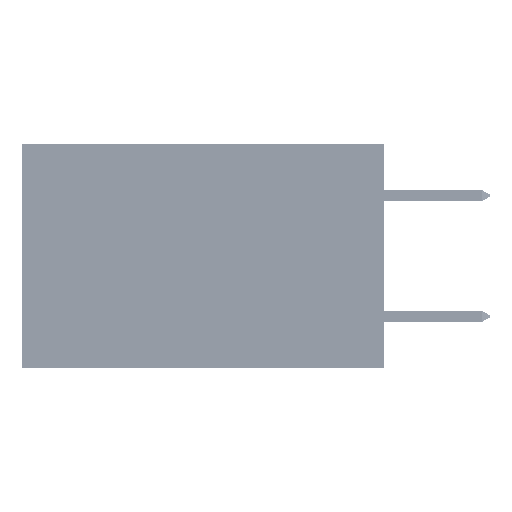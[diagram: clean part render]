
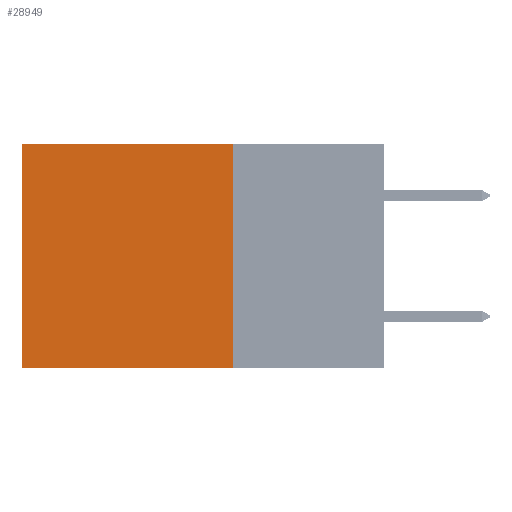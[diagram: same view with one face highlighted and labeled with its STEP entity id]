
A CAD part, left-side view. The second image highlights one B-rep face of the part: STEP entity #28949.
In plain terms, the highlighted planar face has unit normal (-1, 0, 0).
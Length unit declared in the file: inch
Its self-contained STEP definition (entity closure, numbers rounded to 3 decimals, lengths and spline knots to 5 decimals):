
#230 = VERTEX_POINT ( 'NONE', #17198 ) ;
#1277 = DIRECTION ( 'NONE',  ( 0., 0., -1. ) ) ;
#2487 = LINE ( 'NONE', #6239, #3672 ) ;
#3648 = VERTEX_POINT ( 'NONE', #31756 ) ;
#3672 = VECTOR ( 'NONE', #28453, 39.37008 ) ;
#4598 = ORIENTED_EDGE ( 'NONE', *, *, #41679, .T. ) ;
#4755 = CARTESIAN_POINT ( 'NONE',  ( 0.2875, 0.25, 0. ) ) ;
#4766 = CARTESIAN_POINT ( 'NONE',  ( 0.2875, 0.25, -0.37 ) ) ;
#5848 = ORIENTED_EDGE ( 'NONE', *, *, #42059, .F. ) ;
#5929 = LINE ( 'NONE', #4766, #42595 ) ;
#6239 = CARTESIAN_POINT ( 'NONE',  ( 0.2875, 0.6, 0. ) ) ;
#8526 = DIRECTION ( 'NONE',  ( 0., 1., 0. ) ) ;
#9121 = EDGE_LOOP ( 'NONE', ( #4598, #5848, #10436, #25314 ) ) ;
#10164 = LINE ( 'NONE', #4755, #21239 ) ;
#10436 = ORIENTED_EDGE ( 'NONE', *, *, #40183, .F. ) ;
#11801 = AXIS2_PLACEMENT_3D ( 'NONE', #16117, #23579, #1277 ) ;
#15998 = EDGE_CURVE ( 'NONE', #230, #27271, #42469, .T. ) ;
#16117 = CARTESIAN_POINT ( 'NONE',  ( 0.2875, 0.25, 0. ) ) ;
#17198 = CARTESIAN_POINT ( 'NONE',  ( 0.2875, 0.25, 0. ) ) ;
#21239 = VECTOR ( 'NONE', #26979, 39.37008 ) ;
#22643 = DIRECTION ( 'NONE',  ( 0., 1., 0. ) ) ;
#23579 = DIRECTION ( 'NONE',  ( 1., 0., 0. ) ) ;
#25314 = ORIENTED_EDGE ( 'NONE', *, *, #15998, .T. ) ;
#25618 = CARTESIAN_POINT ( 'NONE',  ( 0.2875, 0.6, 0. ) ) ;
#26979 = DIRECTION ( 'NONE',  ( 0., 0., -1. ) ) ;
#27156 = VERTEX_POINT ( 'NONE', #40719 ) ;
#27271 = VERTEX_POINT ( 'NONE', #25618 ) ;
#28453 = DIRECTION ( 'NONE',  ( 0., 0., -1. ) ) ;
#28949 = ADVANCED_FACE ( 'NONE', ( #36743 ), #45067, .F. ) ;
#31756 = CARTESIAN_POINT ( 'NONE',  ( 0.2875, 0.25, -0.37 ) ) ;
#36743 = FACE_OUTER_BOUND ( 'NONE', #9121, .T. ) ;
#40183 = EDGE_CURVE ( 'NONE', #230, #3648, #10164, .T. ) ;
#40628 = CARTESIAN_POINT ( 'NONE',  ( 0.2875, 0.25, 0. ) ) ;
#40719 = CARTESIAN_POINT ( 'NONE',  ( 0.2875, 0.6, -0.37 ) ) ;
#41679 = EDGE_CURVE ( 'NONE', #27271, #27156, #2487, .T. ) ;
#42059 = EDGE_CURVE ( 'NONE', #3648, #27156, #5929, .T. ) ;
#42469 = LINE ( 'NONE', #40628, #43567 ) ;
#42595 = VECTOR ( 'NONE', #8526, 39.37008 ) ;
#43567 = VECTOR ( 'NONE', #22643, 39.37008 ) ;
#45067 = PLANE ( 'NONE',  #11801 ) ;
